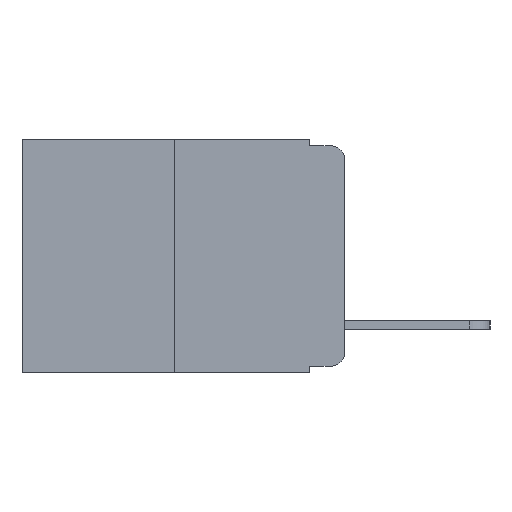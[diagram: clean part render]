
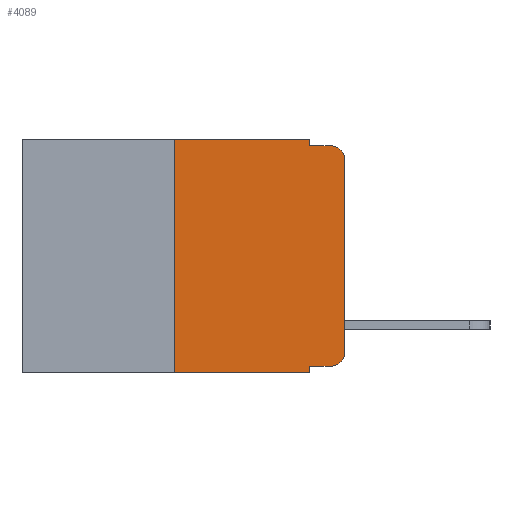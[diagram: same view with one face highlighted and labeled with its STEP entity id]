
A CAD part, left-side view. The second image highlights one B-rep face of the part: STEP entity #4089.
In plain terms, the highlighted planar face has unit normal (-1, 0, 0).
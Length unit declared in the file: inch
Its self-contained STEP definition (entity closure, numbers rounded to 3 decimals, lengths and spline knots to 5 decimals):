
#132 = CARTESIAN_POINT ( 'NONE',  ( 0., 0., 0. ) ) ;
#230 = ORIENTED_EDGE ( 'NONE', *, *, #4960, .F. ) ;
#369 = CARTESIAN_POINT ( 'NONE',  ( 0., 0.051, -0.333 ) ) ;
#458 = ORIENTED_EDGE ( 'NONE', *, *, #4998, .T. ) ;
#474 = ORIENTED_EDGE ( 'NONE', *, *, #4938, .T. ) ;
#560 = FACE_OUTER_BOUND ( 'NONE', #2842, .T. ) ;
#901 = LINE ( 'NONE', #6046, #6246 ) ;
#1231 = DIRECTION ( 'NONE',  ( 0., 0., -1. ) ) ;
#1418 = DIRECTION ( 'NONE',  ( 1., 0., 0. ) ) ;
#1847 = VERTEX_POINT ( 'NONE', #2541 ) ;
#1906 = AXIS2_PLACEMENT_3D ( 'NONE', #6481, #4551, #4599 ) ;
#2039 = CARTESIAN_POINT ( 'NONE',  ( 0., 0., -0.313 ) ) ;
#2073 = AXIS2_PLACEMENT_3D ( 'NONE', #2735, #2638, #11441 ) ;
#2118 = CARTESIAN_POINT ( 'NONE',  ( 0., 0.051, 0. ) ) ;
#2322 = VECTOR ( 'NONE', #11674, 39.37008 ) ;
#2354 = CARTESIAN_POINT ( 'NONE',  ( 0., 0., -0.03 ) ) ;
#2541 = CARTESIAN_POINT ( 'NONE',  ( 0., 0.02, -0.333 ) ) ;
#2638 = DIRECTION ( 'NONE',  ( -1., 0., 0. ) ) ;
#2735 = CARTESIAN_POINT ( 'NONE',  ( 0., 0.02, -0.03 ) ) ;
#2842 = EDGE_LOOP ( 'NONE', ( #474, #6385, #230, #4535, #4140, #3484, #5800, #5645, #9136, #458 ) ) ;
#3404 = VERTEX_POINT ( 'NONE', #5999 ) ;
#3458 = CARTESIAN_POINT ( 'NONE',  ( 0., 0.25, 0. ) ) ;
#3484 = ORIENTED_EDGE ( 'NONE', *, *, #4977, .F. ) ;
#3549 = CARTESIAN_POINT ( 'NONE',  ( 0., 0.051, 0. ) ) ;
#3572 = DIRECTION ( 'NONE',  ( 0., -1., 0. ) ) ;
#3601 = DIRECTION ( 'NONE',  ( 0., 0., 1. ) ) ;
#4089 = ADVANCED_FACE ( 'NONE', ( #560 ), #9887, .F. ) ;
#4140 = ORIENTED_EDGE ( 'NONE', *, *, #4499, .F. ) ;
#4188 = VECTOR ( 'NONE', #11007, 39.37008 ) ;
#4199 = LINE ( 'NONE', #6578, #6496 ) ;
#4452 = DIRECTION ( 'NONE',  ( 0., -1., 0. ) ) ;
#4499 = EDGE_CURVE ( 'NONE', #4825, #4849, #4863, .T. ) ;
#4535 = ORIENTED_EDGE ( 'NONE', *, *, #4963, .F. ) ;
#4551 = DIRECTION ( 'NONE',  ( -1., 0., 0. ) ) ;
#4599 = DIRECTION ( 'NONE',  ( 0., 0., -1. ) ) ;
#4772 = EDGE_CURVE ( 'NONE', #5541, #8927, #4199, .T. ) ;
#4825 = VERTEX_POINT ( 'NONE', #3458 ) ;
#4831 = LINE ( 'NONE', #3549, #4188 ) ;
#4849 = VERTEX_POINT ( 'NONE', #11051 ) ;
#4863 = LINE ( 'NONE', #6602, #11202 ) ;
#4938 = EDGE_CURVE ( 'NONE', #6609, #5904, #9694, .T. ) ;
#4940 = EDGE_CURVE ( 'NONE', #5904, #3404, #5176, .T. ) ;
#4960 = EDGE_CURVE ( 'NONE', #7525, #3404, #11182, .T. ) ;
#4963 = EDGE_CURVE ( 'NONE', #4849, #7525, #4831, .T. ) ;
#4977 = EDGE_CURVE ( 'NONE', #5541, #4825, #8734, .T. ) ;
#4980 = EDGE_CURVE ( 'NONE', #9595, #8927, #8982, .T. ) ;
#4981 = EDGE_CURVE ( 'NONE', #9595, #1847, #901, .T. ) ;
#4998 = EDGE_CURVE ( 'NONE', #1847, #6609, #10248, .T. ) ;
#5176 = CIRCLE ( 'NONE', #2073, 0.02 ) ;
#5541 = VERTEX_POINT ( 'NONE', #8980 ) ;
#5645 = ORIENTED_EDGE ( 'NONE', *, *, #4980, .F. ) ;
#5800 = ORIENTED_EDGE ( 'NONE', *, *, #4772, .T. ) ;
#5904 = VERTEX_POINT ( 'NONE', #2354 ) ;
#5999 = CARTESIAN_POINT ( 'NONE',  ( 0., 0.02, -0.01 ) ) ;
#6046 = CARTESIAN_POINT ( 'NONE',  ( 0., 0.051, -0.333 ) ) ;
#6246 = VECTOR ( 'NONE', #6665, 39.37008 ) ;
#6385 = ORIENTED_EDGE ( 'NONE', *, *, #4940, .T. ) ;
#6481 = CARTESIAN_POINT ( 'NONE',  ( 0., 0.02, -0.313 ) ) ;
#6496 = VECTOR ( 'NONE', #4452, 39.37008 ) ;
#6578 = CARTESIAN_POINT ( 'NONE',  ( 0., 0.473, -0.343 ) ) ;
#6602 = CARTESIAN_POINT ( 'NONE',  ( 0., 0.473, 0. ) ) ;
#6609 = VERTEX_POINT ( 'NONE', #2039 ) ;
#6665 = DIRECTION ( 'NONE',  ( 0., -1., 0. ) ) ;
#6731 = VECTOR ( 'NONE', #3601, 39.37008 ) ;
#6752 = CARTESIAN_POINT ( 'NONE',  ( 0., 0.051, -0.343 ) ) ;
#7525 = VERTEX_POINT ( 'NONE', #7708 ) ;
#7708 = CARTESIAN_POINT ( 'NONE',  ( 0., 0.051, -0.01 ) ) ;
#7926 = CARTESIAN_POINT ( 'NONE',  ( 0., 0.051, -0.01 ) ) ;
#7954 = DIRECTION ( 'NONE',  ( 0., 0., -1. ) ) ;
#8175 = AXIS2_PLACEMENT_3D ( 'NONE', #10564, #1418, #1231 ) ;
#8406 = CARTESIAN_POINT ( 'NONE',  ( 0., 0.25, 0. ) ) ;
#8734 = LINE ( 'NONE', #8406, #6731 ) ;
#8927 = VERTEX_POINT ( 'NONE', #6752 ) ;
#8980 = CARTESIAN_POINT ( 'NONE',  ( 0., 0.25, -0.343 ) ) ;
#8982 = LINE ( 'NONE', #2118, #10501 ) ;
#9136 = ORIENTED_EDGE ( 'NONE', *, *, #4981, .T. ) ;
#9595 = VERTEX_POINT ( 'NONE', #369 ) ;
#9694 = LINE ( 'NONE', #132, #2322 ) ;
#9887 = PLANE ( 'NONE',  #8175 ) ;
#10248 = CIRCLE ( 'NONE', #1906, 0.02 ) ;
#10501 = VECTOR ( 'NONE', #7954, 39.37008 ) ;
#10564 = CARTESIAN_POINT ( 'NONE',  ( 0., 0.473, 0. ) ) ;
#10952 = VECTOR ( 'NONE', #3572, 39.37008 ) ;
#11007 = DIRECTION ( 'NONE',  ( 0., 0., -1. ) ) ;
#11051 = CARTESIAN_POINT ( 'NONE',  ( 0., 0.051, 0. ) ) ;
#11182 = LINE ( 'NONE', #7926, #10952 ) ;
#11202 = VECTOR ( 'NONE', #11472, 39.37008 ) ;
#11441 = DIRECTION ( 'NONE',  ( 0., 0., -1. ) ) ;
#11472 = DIRECTION ( 'NONE',  ( 0., -1., 0. ) ) ;
#11674 = DIRECTION ( 'NONE',  ( 0., 0., 1. ) ) ;
